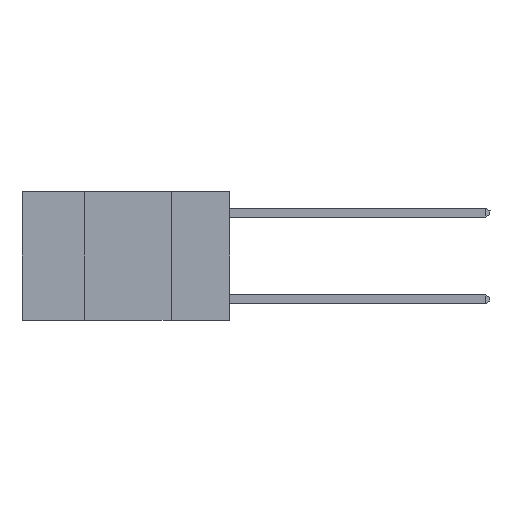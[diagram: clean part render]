
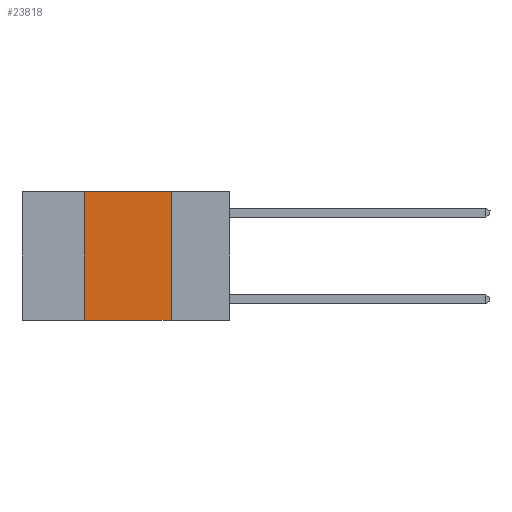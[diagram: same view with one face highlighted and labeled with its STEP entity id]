
A CAD part, left-side view. The second image highlights one B-rep face of the part: STEP entity #23818.
In plain terms, the highlighted planar face has unit normal (-1, 0, 0).
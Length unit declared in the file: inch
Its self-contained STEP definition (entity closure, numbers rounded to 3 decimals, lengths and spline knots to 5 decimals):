
#803 = DIRECTION ( 'NONE',  ( 0., 0., -1. ) ) ;
#2895 = CARTESIAN_POINT ( 'NONE',  ( 0., 0.6, 0. ) ) ;
#3791 = LINE ( 'NONE', #13367, #25924 ) ;
#4226 = LINE ( 'NONE', #11622, #9282 ) ;
#4286 = EDGE_CURVE ( 'NONE', #23199, #27180, #11295, .T. ) ;
#4652 = VERTEX_POINT ( 'NONE', #25371 ) ;
#4670 = VECTOR ( 'NONE', #12889, 39.37008 ) ;
#5092 = EDGE_CURVE ( 'NONE', #27180, #4652, #4226, .T. ) ;
#5478 = EDGE_LOOP ( 'NONE', ( #16921, #21120, #17517, #17381 ) ) ;
#5562 = FACE_OUTER_BOUND ( 'NONE', #5478, .T. ) ;
#5792 = DIRECTION ( 'NONE',  ( 1., 0., 0. ) ) ;
#6935 = VECTOR ( 'NONE', #9306, 39.37008 ) ;
#7872 = PLANE ( 'NONE',  #8429 ) ;
#8429 = AXIS2_PLACEMENT_3D ( 'NONE', #18655, #5792, #20799 ) ;
#9255 = EDGE_CURVE ( 'NONE', #25378, #23199, #26110, .T. ) ;
#9282 = VECTOR ( 'NONE', #803, 39.37008 ) ;
#9306 = DIRECTION ( 'NONE',  ( 0., -1., 0. ) ) ;
#11295 = LINE ( 'NONE', #2895, #6935 ) ;
#11622 = CARTESIAN_POINT ( 'NONE',  ( 0., 0.17, 0. ) ) ;
#12398 = CARTESIAN_POINT ( 'NONE',  ( 0., 0.42, 0. ) ) ;
#12889 = DIRECTION ( 'NONE',  ( 0., 0., 1. ) ) ;
#13367 = CARTESIAN_POINT ( 'NONE',  ( 0., 0.6, -0.37 ) ) ;
#15551 = DIRECTION ( 'NONE',  ( 0., -1., 0. ) ) ;
#16470 = CARTESIAN_POINT ( 'NONE',  ( 0., 0.17, 0. ) ) ;
#16921 = ORIENTED_EDGE ( 'NONE', *, *, #5092, .F. ) ;
#17381 = ORIENTED_EDGE ( 'NONE', *, *, #22835, .T. ) ;
#17517 = ORIENTED_EDGE ( 'NONE', *, *, #9255, .F. ) ;
#18655 = CARTESIAN_POINT ( 'NONE',  ( 0., 0.6, 0. ) ) ;
#20799 = DIRECTION ( 'NONE',  ( 0., 0., -1. ) ) ;
#21120 = ORIENTED_EDGE ( 'NONE', *, *, #4286, .F. ) ;
#22835 = EDGE_CURVE ( 'NONE', #25378, #4652, #3791, .T. ) ;
#23199 = VERTEX_POINT ( 'NONE', #12398 ) ;
#23818 = ADVANCED_FACE ( 'NONE', ( #5562 ), #7872, .F. ) ;
#25371 = CARTESIAN_POINT ( 'NONE',  ( 0., 0.17, -0.37 ) ) ;
#25378 = VERTEX_POINT ( 'NONE', #27060 ) ;
#25671 = CARTESIAN_POINT ( 'NONE',  ( 0., 0.42, 0. ) ) ;
#25924 = VECTOR ( 'NONE', #15551, 39.37008 ) ;
#26110 = LINE ( 'NONE', #25671, #4670 ) ;
#27060 = CARTESIAN_POINT ( 'NONE',  ( 0., 0.42, -0.37 ) ) ;
#27180 = VERTEX_POINT ( 'NONE', #16470 ) ;
